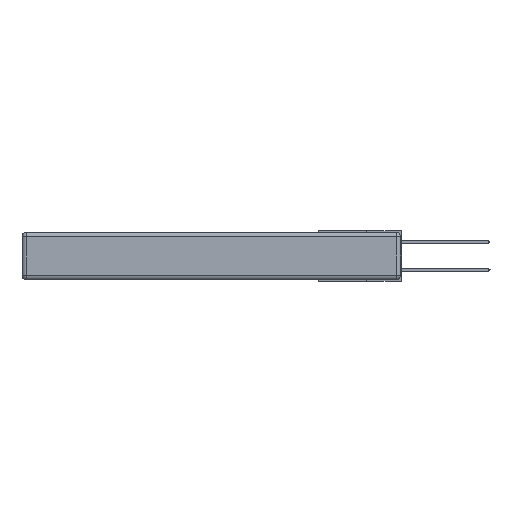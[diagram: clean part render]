
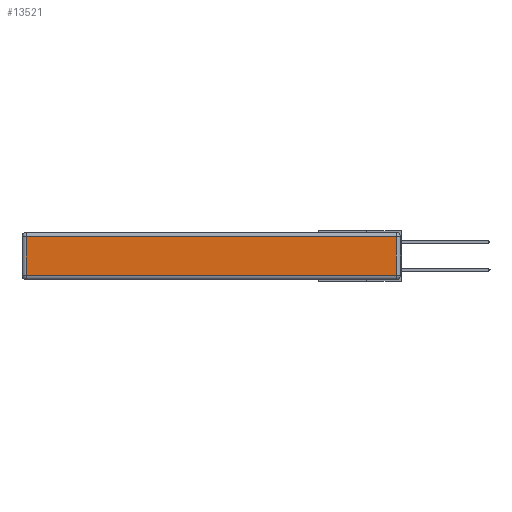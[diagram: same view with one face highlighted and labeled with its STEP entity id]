
A CAD part, left-side view. The second image highlights one B-rep face of the part: STEP entity #13521.
In plain terms, the highlighted planar face has unit normal (-1, 0, 0).
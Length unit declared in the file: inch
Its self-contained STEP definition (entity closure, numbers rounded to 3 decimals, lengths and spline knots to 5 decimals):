
#370 = CARTESIAN_POINT ( 'NONE',  ( 0., 2.75, -0.03 ) ) ;
#922 = AXIS2_PLACEMENT_3D ( 'NONE', #18246, #20328, #14674 ) ;
#2448 = LINE ( 'NONE', #9540, #15948 ) ;
#3579 = DIRECTION ( 'NONE',  ( 0., -1., 0. ) ) ;
#3929 = ORIENTED_EDGE ( 'NONE', *, *, #14153, .T. ) ;
#4299 = VERTEX_POINT ( 'NONE', #13563 ) ;
#4386 = LINE ( 'NONE', #21632, #22995 ) ;
#5008 = VERTEX_POINT ( 'NONE', #6172 ) ;
#5743 = EDGE_CURVE ( 'NONE', #4299, #11689, #16835, .T. ) ;
#6172 = CARTESIAN_POINT ( 'NONE',  ( 0., 0.03, -0.313 ) ) ;
#6381 = DIRECTION ( 'NONE',  ( 0., 1., 0. ) ) ;
#6637 = EDGE_CURVE ( 'NONE', #16086, #5008, #9009, .T. ) ;
#6789 = FACE_OUTER_BOUND ( 'NONE', #11850, .T. ) ;
#7119 = CARTESIAN_POINT ( 'NONE',  ( 0., 0., -0.313 ) ) ;
#9009 = LINE ( 'NONE', #7119, #11867 ) ;
#9540 = CARTESIAN_POINT ( 'NONE',  ( 0., 0.03, -0.343 ) ) ;
#9654 = ORIENTED_EDGE ( 'NONE', *, *, #21305, .T. ) ;
#10745 = VECTOR ( 'NONE', #6381, 39.37008 ) ;
#11442 = ORIENTED_EDGE ( 'NONE', *, *, #5743, .T. ) ;
#11689 = VERTEX_POINT ( 'NONE', #22325 ) ;
#11850 = EDGE_LOOP ( 'NONE', ( #23210, #3929, #11442, #9654 ) ) ;
#11867 = VECTOR ( 'NONE', #3579, 39.37008 ) ;
#13521 = ADVANCED_FACE ( 'NONE', ( #6789 ), #23625, .T. ) ;
#13563 = CARTESIAN_POINT ( 'NONE',  ( 0., 0.03, -0.03 ) ) ;
#13951 = CARTESIAN_POINT ( 'NONE',  ( 0., 2.72, -0.313 ) ) ;
#14153 = EDGE_CURVE ( 'NONE', #5008, #4299, #2448, .T. ) ;
#14159 = DIRECTION ( 'NONE',  ( 0., 0., -1. ) ) ;
#14674 = DIRECTION ( 'NONE',  ( 0., 0., 1. ) ) ;
#15948 = VECTOR ( 'NONE', #23115, 39.37008 ) ;
#16086 = VERTEX_POINT ( 'NONE', #13951 ) ;
#16835 = LINE ( 'NONE', #370, #10745 ) ;
#18246 = CARTESIAN_POINT ( 'NONE',  ( 0., 0., -0.343 ) ) ;
#20328 = DIRECTION ( 'NONE',  ( -1., 0., 0. ) ) ;
#21305 = EDGE_CURVE ( 'NONE', #11689, #16086, #4386, .T. ) ;
#21632 = CARTESIAN_POINT ( 'NONE',  ( 0., 2.72, -0.343 ) ) ;
#22325 = CARTESIAN_POINT ( 'NONE',  ( 0., 2.72, -0.03 ) ) ;
#22995 = VECTOR ( 'NONE', #14159, 39.37008 ) ;
#23115 = DIRECTION ( 'NONE',  ( 0., 0., 1. ) ) ;
#23210 = ORIENTED_EDGE ( 'NONE', *, *, #6637, .T. ) ;
#23625 = PLANE ( 'NONE',  #922 ) ;
